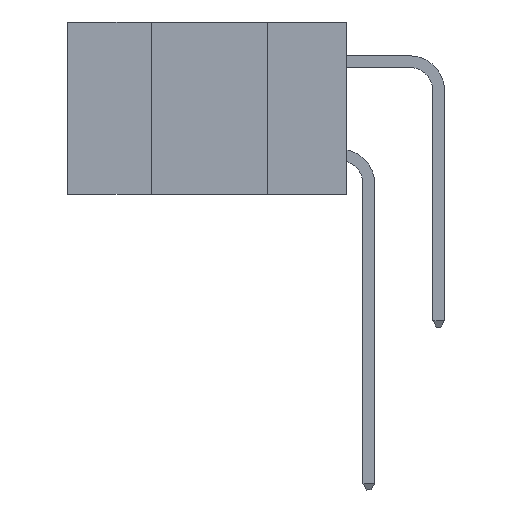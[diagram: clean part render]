
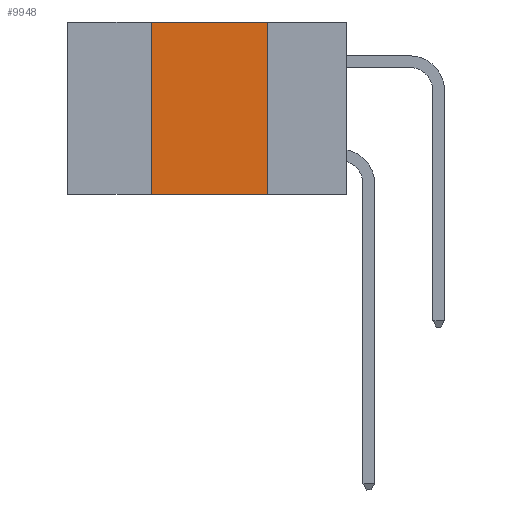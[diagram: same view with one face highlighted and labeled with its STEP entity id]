
A CAD part, left-side view. The second image highlights one B-rep face of the part: STEP entity #9948.
In plain terms, the highlighted planar face has unit normal (-1, 0, 0).
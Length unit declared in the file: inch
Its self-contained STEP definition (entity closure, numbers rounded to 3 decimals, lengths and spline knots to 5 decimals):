
#861 = LINE ( 'NONE', #3459, #7367 ) ;
#1361 = CARTESIAN_POINT ( 'NONE',  ( 0., 0.42, -0.37 ) ) ;
#1850 = PLANE ( 'NONE',  #7606 ) ;
#1878 = CARTESIAN_POINT ( 'NONE',  ( 0., 0.17, -0.37 ) ) ;
#2746 = EDGE_CURVE ( 'NONE', #8366, #15991, #6542, .T. ) ;
#3031 = LINE ( 'NONE', #5704, #13322 ) ;
#3459 = CARTESIAN_POINT ( 'NONE',  ( 0., 0.17, 0. ) ) ;
#3723 = DIRECTION ( 'NONE',  ( 0., 0., -1. ) ) ;
#4291 = LINE ( 'NONE', #15750, #7780 ) ;
#5462 = CARTESIAN_POINT ( 'NONE',  ( 0., 0.42, 0. ) ) ;
#5704 = CARTESIAN_POINT ( 'NONE',  ( 0., 0.6, -0.37 ) ) ;
#5732 = CARTESIAN_POINT ( 'NONE',  ( 0., 0.6, 0. ) ) ;
#6542 = LINE ( 'NONE', #10655, #16115 ) ;
#6826 = EDGE_CURVE ( 'NONE', #13882, #15421, #861, .T. ) ;
#6853 = ORIENTED_EDGE ( 'NONE', *, *, #2746, .F. ) ;
#7068 = DIRECTION ( 'NONE',  ( 0., 0., -1. ) ) ;
#7367 = VECTOR ( 'NONE', #3723, 39.37008 ) ;
#7494 = ORIENTED_EDGE ( 'NONE', *, *, #13548, .F. ) ;
#7606 = AXIS2_PLACEMENT_3D ( 'NONE', #5732, #14703, #7068 ) ;
#7780 = VECTOR ( 'NONE', #13245, 39.37008 ) ;
#8366 = VERTEX_POINT ( 'NONE', #1361 ) ;
#8716 = FACE_OUTER_BOUND ( 'NONE', #14701, .T. ) ;
#9948 = ADVANCED_FACE ( 'NONE', ( #8716 ), #1850, .F. ) ;
#10655 = CARTESIAN_POINT ( 'NONE',  ( 0., 0.42, 0. ) ) ;
#10721 = ORIENTED_EDGE ( 'NONE', *, *, #6826, .F. ) ;
#10988 = DIRECTION ( 'NONE',  ( 0., 0., 1. ) ) ;
#13245 = DIRECTION ( 'NONE',  ( 0., -1., 0. ) ) ;
#13322 = VECTOR ( 'NONE', #13410, 39.37008 ) ;
#13410 = DIRECTION ( 'NONE',  ( 0., -1., 0. ) ) ;
#13472 = ORIENTED_EDGE ( 'NONE', *, *, #13629, .T. ) ;
#13548 = EDGE_CURVE ( 'NONE', #15991, #13882, #4291, .T. ) ;
#13629 = EDGE_CURVE ( 'NONE', #8366, #15421, #3031, .T. ) ;
#13882 = VERTEX_POINT ( 'NONE', #15142 ) ;
#14701 = EDGE_LOOP ( 'NONE', ( #10721, #7494, #6853, #13472 ) ) ;
#14703 = DIRECTION ( 'NONE',  ( 1., 0., 0. ) ) ;
#15142 = CARTESIAN_POINT ( 'NONE',  ( 0., 0.17, 0. ) ) ;
#15421 = VERTEX_POINT ( 'NONE', #1878 ) ;
#15750 = CARTESIAN_POINT ( 'NONE',  ( 0., 0.6, 0. ) ) ;
#15991 = VERTEX_POINT ( 'NONE', #5462 ) ;
#16115 = VECTOR ( 'NONE', #10988, 39.37008 ) ;
